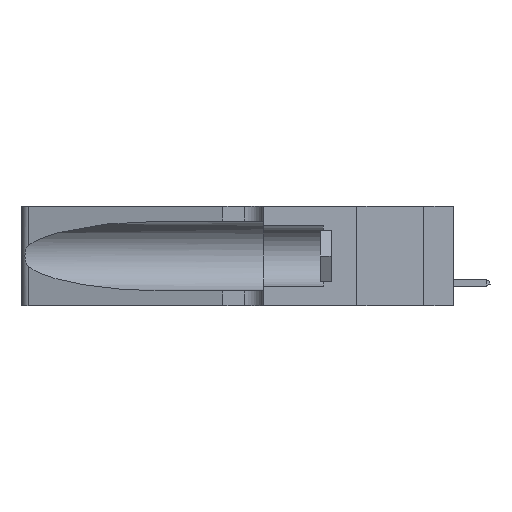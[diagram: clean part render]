
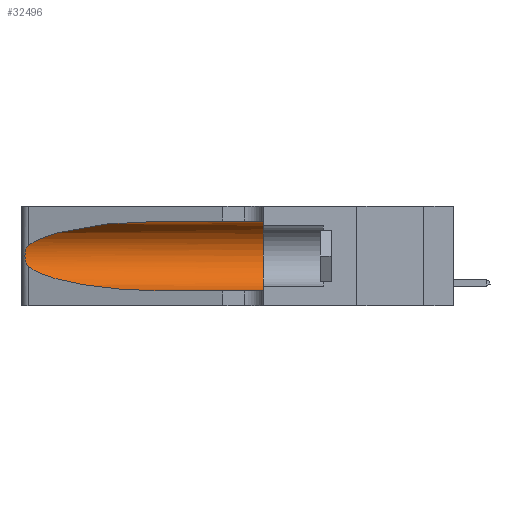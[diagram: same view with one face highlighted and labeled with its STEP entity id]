
A CAD part, left-side view. The second image highlights one B-rep face of the part: STEP entity #32496.
In plain terms, the highlighted cylindrical face has radius 3.308 mm (diameter 6.617 mm), a partial arc.
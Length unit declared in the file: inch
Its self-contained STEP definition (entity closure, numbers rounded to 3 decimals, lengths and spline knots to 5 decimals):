
#526 = CARTESIAN_POINT ( 'NONE',  ( 0.2373, 1.15595, 0.08982 ) ) ;
#540 = EDGE_CURVE ( 'NONE', #25988, #24471, #23048, .T. ) ;
#1083 = EDGE_CURVE ( 'NONE', #32954, #16823, #8015, .T. ) ;
#2139 = LINE ( 'NONE', #17472, #17869 ) ;
#2849 = CARTESIAN_POINT ( 'NONE',  ( 0.25787, 1.23484, 0.2124 ) ) ;
#3522 = DIRECTION ( 'NONE',  ( 0., -1., 0. ) ) ;
#3672 = CARTESIAN_POINT ( 'NONE',  ( 0.25639, 1.23184, 0.21858 ) ) ;
#3986 = CARTESIAN_POINT ( 'NONE',  ( 0.1305, 0.72297, 0.05475 ) ) ;
#4405 = CYLINDRICAL_SURFACE ( 'NONE', #36331, 0.13025 ) ;
#4905 =( BOUNDED_CURVE ( )  B_SPLINE_CURVE ( 3, ( #12363, #26245, #26383, #18274 ),
 .UNSPECIFIED., .F., .T. ) 
 B_SPLINE_CURVE_WITH_KNOTS ( ( 4, 4 ),
 ( 1.5708, 2.84003 ),
 .UNSPECIFIED. ) 
 CURVE ( )  GEOMETRIC_REPRESENTATION_ITEM ( )  RATIONAL_B_SPLINE_CURVE ( ( 1., 0.87, 0.87, 1. ) ) 
 REPRESENTATION_ITEM ( '' )  );
#5065 =( BOUNDED_CURVE ( )  B_SPLINE_CURVE ( 3, ( #33715, #526, #22814, #14142 ),
 .UNSPECIFIED., .F., .T. ) 
 B_SPLINE_CURVE_WITH_KNOTS ( ( 4, 4 ),
 ( 3.44316, 4.71239 ),
 .UNSPECIFIED. ) 
 CURVE ( )  GEOMETRIC_REPRESENTATION_ITEM ( )  RATIONAL_B_SPLINE_CURVE ( ( 1., 0.87, 0.87, 1. ) ) 
 REPRESENTATION_ITEM ( '' )  );
#5639 = EDGE_CURVE ( 'NONE', #24471, #27849, #26921, .T. ) ;
#6213 = CARTESIAN_POINT ( 'NONE',  ( 0.1305, 0.35, 0.185 ) ) ;
#8015 = B_SPLINE_CURVE_WITH_KNOTS ( 'NONE', 3,
 ( #19061, #16780, #3672, #2849, #22822, #34438, #20131, #22949, #9084, #31755, #20266, #23074, #17565, #21204 ),
 .UNSPECIFIED., .F., .F.,
 ( 4, 2, 2, 2, 2, 2, 4 ),
 ( 0., 0.00027, 0.00053, 0.00107, 0.0016, 0.00187, 0.00214 ),
 .UNSPECIFIED. ) ;
#9084 = CARTESIAN_POINT ( 'NONE',  ( 0.26017, 1.23833, 0.17102 ) ) ;
#9335 = CARTESIAN_POINT ( 'NONE',  ( 0.1305, 0.35, 0.31525 ) ) ;
#9752 = ORIENTED_EDGE ( 'NONE', *, *, #1083, .T. ) ;
#10468 = DIRECTION ( 'NONE',  ( 0., -1., 0. ) ) ;
#12363 = CARTESIAN_POINT ( 'NONE',  ( 0.1305, 0.72297, 0.31525 ) ) ;
#12617 = EDGE_CURVE ( 'NONE', #21008, #27849, #2139, .T. ) ;
#12976 = EDGE_LOOP ( 'NONE', ( #34245, #9752, #31673, #33857, #21390, #14331 ) ) ;
#14142 = CARTESIAN_POINT ( 'NONE',  ( 0.1305, 0.72297, 0.05475 ) ) ;
#14331 = ORIENTED_EDGE ( 'NONE', *, *, #540, .F. ) ;
#16780 = CARTESIAN_POINT ( 'NONE',  ( 0.25555, 1.22994, 0.2215 ) ) ;
#16823 = VERTEX_POINT ( 'NONE', #34365 ) ;
#17472 = CARTESIAN_POINT ( 'NONE',  ( 0.1305, 1.61858, 0.05475 ) ) ;
#17522 = EDGE_CURVE ( 'NONE', #25988, #32954, #4905, .T. ) ;
#17565 = CARTESIAN_POINT ( 'NONE',  ( 0.25555, 1.22993, 0.14849 ) ) ;
#17869 = VECTOR ( 'NONE', #34483, 39.37008 ) ;
#18235 = CARTESIAN_POINT ( 'NONE',  ( 0.1305, 1.61858, 0.31525 ) ) ;
#18274 = CARTESIAN_POINT ( 'NONE',  ( 0.25487, 1.22718, 0.22369 ) ) ;
#19061 = CARTESIAN_POINT ( 'NONE',  ( 0.25487, 1.22718, 0.22369 ) ) ;
#20131 = CARTESIAN_POINT ( 'NONE',  ( 0.26075, 1.23896, 0.19203 ) ) ;
#20266 = CARTESIAN_POINT ( 'NONE',  ( 0.25789, 1.23486, 0.15765 ) ) ;
#21008 = VERTEX_POINT ( 'NONE', #3986 ) ;
#21204 = CARTESIAN_POINT ( 'NONE',  ( 0.25487, 1.22718, 0.14631 ) ) ;
#21289 = CARTESIAN_POINT ( 'NONE',  ( 0.1305, 0.72297, 0.31525 ) ) ;
#21390 = ORIENTED_EDGE ( 'NONE', *, *, #5639, .F. ) ;
#22814 = CARTESIAN_POINT ( 'NONE',  ( 0.18966, 0.96281, 0.05475 ) ) ;
#22822 = CARTESIAN_POINT ( 'NONE',  ( 0.25854, 1.2359, 0.20912 ) ) ;
#22949 = CARTESIAN_POINT ( 'NONE',  ( 0.26075, 1.23896, 0.178 ) ) ;
#23048 = LINE ( 'NONE', #18235, #30986 ) ;
#23074 = CARTESIAN_POINT ( 'NONE',  ( 0.25639, 1.23186, 0.15144 ) ) ;
#24471 = VERTEX_POINT ( 'NONE', #9335 ) ;
#25988 = VERTEX_POINT ( 'NONE', #21289 ) ;
#26245 = CARTESIAN_POINT ( 'NONE',  ( 0.18966, 0.96281, 0.31525 ) ) ;
#26348 = DIRECTION ( 'NONE',  ( 0., 0., 1. ) ) ;
#26383 = CARTESIAN_POINT ( 'NONE',  ( 0.2373, 1.15595, 0.28018 ) ) ;
#26921 = CIRCLE ( 'NONE', #33006, 0.13025 ) ;
#27184 = FACE_OUTER_BOUND ( 'NONE', #12976, .T. ) ;
#27265 = CARTESIAN_POINT ( 'NONE',  ( 0.25487, 1.22718, 0.22369 ) ) ;
#27849 = VERTEX_POINT ( 'NONE', #28536 ) ;
#28536 = CARTESIAN_POINT ( 'NONE',  ( 0.1305, 0.35, 0.05475 ) ) ;
#28801 = DIRECTION ( 'NONE',  ( 0., 1., 0. ) ) ;
#30147 = DIRECTION ( 'NONE',  ( 0., 0., -1. ) ) ;
#30358 = EDGE_CURVE ( 'NONE', #16823, #21008, #5065, .T. ) ;
#30986 = VECTOR ( 'NONE', #3522, 39.37008 ) ;
#31673 = ORIENTED_EDGE ( 'NONE', *, *, #30358, .T. ) ;
#31755 = CARTESIAN_POINT ( 'NONE',  ( 0.25856, 1.23593, 0.16098 ) ) ;
#32496 = ADVANCED_FACE ( 'NONE', ( #27184 ), #4405, .F. ) ;
#32954 = VERTEX_POINT ( 'NONE', #27265 ) ;
#33006 = AXIS2_PLACEMENT_3D ( 'NONE', #6213, #28801, #26348 ) ;
#33715 = CARTESIAN_POINT ( 'NONE',  ( 0.25487, 1.22718, 0.14631 ) ) ;
#33857 = ORIENTED_EDGE ( 'NONE', *, *, #12617, .T. ) ;
#34245 = ORIENTED_EDGE ( 'NONE', *, *, #17522, .T. ) ;
#34365 = CARTESIAN_POINT ( 'NONE',  ( 0.25487, 1.22718, 0.14631 ) ) ;
#34438 = CARTESIAN_POINT ( 'NONE',  ( 0.26018, 1.23835, 0.19895 ) ) ;
#34483 = DIRECTION ( 'NONE',  ( 0., -1., 0. ) ) ;
#35942 = CARTESIAN_POINT ( 'NONE',  ( 0.1305, 1.61858, 0.185 ) ) ;
#36331 = AXIS2_PLACEMENT_3D ( 'NONE', #35942, #10468, #30147 ) ;
